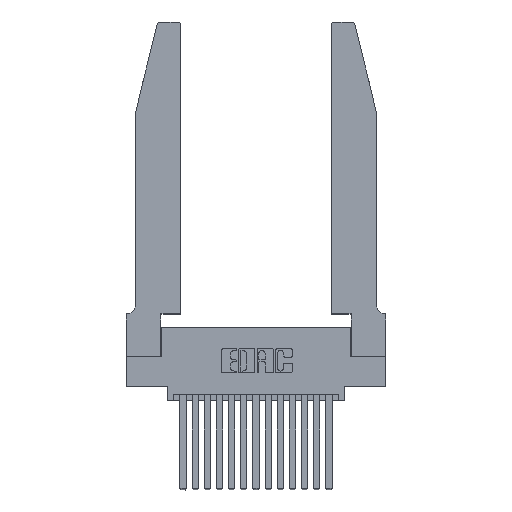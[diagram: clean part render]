
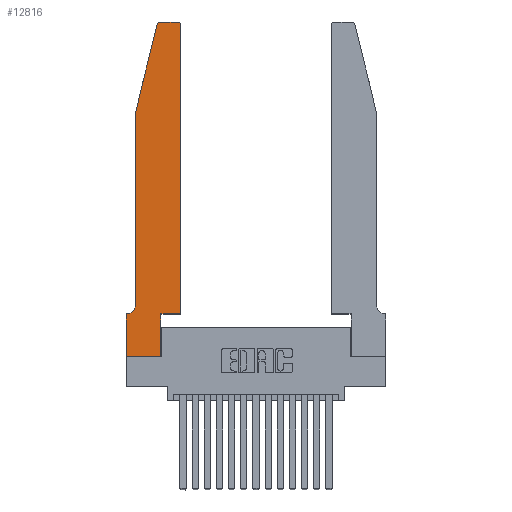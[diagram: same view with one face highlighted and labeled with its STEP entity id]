
A CAD part, top view. The second image highlights one B-rep face of the part: STEP entity #12816.
In plain terms, the highlighted planar face has unit normal (0, 0, 1).
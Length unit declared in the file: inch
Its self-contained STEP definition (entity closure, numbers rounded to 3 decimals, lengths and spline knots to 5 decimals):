
#47 = ORIENTED_EDGE ( 'NONE', *, *, #8778, .T. ) ;
#226 = LINE ( 'NONE', #14997, #3623 ) ;
#280 = VECTOR ( 'NONE', #14104, 39.37008 ) ;
#457 = DIRECTION ( 'NONE',  ( 0., 1., 0. ) ) ;
#633 = CARTESIAN_POINT ( 'NONE',  ( 0.0755, 0.35, 0.37 ) ) ;
#1047 = DIRECTION ( 'NONE',  ( 1., 0., 0. ) ) ;
#1264 = CARTESIAN_POINT ( 'NONE',  ( 0.0755, 2., 0.37 ) ) ;
#1401 = LINE ( 'NONE', #5710, #7119 ) ;
#1420 = EDGE_CURVE ( 'NONE', #13402, #14783, #5633, .T. ) ;
#1527 = EDGE_CURVE ( 'NONE', #6601, #16850, #15638, .T. ) ;
#1724 = ORIENTED_EDGE ( 'NONE', *, *, #17017, .T. ) ;
#1955 = DIRECTION ( 'NONE',  ( 1., 0., 0. ) ) ;
#2006 = ORIENTED_EDGE ( 'NONE', *, *, #1420, .T. ) ;
#2154 = CARTESIAN_POINT ( 'NONE',  ( 0.0055, 0.42, 0.37 ) ) ;
#2495 = DIRECTION ( 'NONE',  ( -1., 0., 0. ) ) ;
#2535 = AXIS2_PLACEMENT_3D ( 'NONE', #2154, #5106, #16919 ) ;
#2571 = LINE ( 'NONE', #15739, #7391 ) ;
#2753 = EDGE_CURVE ( 'NONE', #9355, #13402, #16266, .T. ) ;
#2881 = DIRECTION ( 'NONE',  ( 0., -1., 0. ) ) ;
#3074 = CARTESIAN_POINT ( 'NONE',  ( 0., 0., 0.37 ) ) ;
#3121 = ORIENTED_EDGE ( 'NONE', *, *, #12940, .T. ) ;
#3542 = DIRECTION ( 'NONE',  ( -1., 0., 0. ) ) ;
#3623 = VECTOR ( 'NONE', #1955, 39.37008 ) ;
#3868 = VERTEX_POINT ( 'NONE', #18828 ) ;
#3893 = CARTESIAN_POINT ( 'NONE',  ( 0., 0.35, 0.37 ) ) ;
#3898 = CARTESIAN_POINT ( 'NONE',  ( 0.0755, 0.42, 0.37 ) ) ;
#3967 = CARTESIAN_POINT ( 'NONE',  ( 0.0755, 2., 0.37 ) ) ;
#4467 = EDGE_CURVE ( 'NONE', #14783, #17610, #13930, .T. ) ;
#4891 = VECTOR ( 'NONE', #10074, 39.37008 ) ;
#5106 = DIRECTION ( 'NONE',  ( 0., 0., -1. ) ) ;
#5339 = CARTESIAN_POINT ( 'NONE',  ( 0.2865, 0.35, 0.37 ) ) ;
#5503 = VERTEX_POINT ( 'NONE', #17672 ) ;
#5603 = CARTESIAN_POINT ( 'NONE',  ( 0.284, 2.72, 0.37 ) ) ;
#5610 = EDGE_CURVE ( 'NONE', #18834, #8121, #226, .T. ) ;
#5633 = CIRCLE ( 'NONE', #2535, 0.07 ) ;
#5706 = DIRECTION ( 'NONE',  ( 0., 0., 1. ) ) ;
#5710 = CARTESIAN_POINT ( 'NONE',  ( 0.4505, 0.35, 0.37 ) ) ;
#6427 = VECTOR ( 'NONE', #3542, 39.37008 ) ;
#6445 = ORIENTED_EDGE ( 'NONE', *, *, #10092, .T. ) ;
#6601 = VERTEX_POINT ( 'NONE', #18458 ) ;
#6983 = PLANE ( 'NONE',  #14503 ) ;
#7119 = VECTOR ( 'NONE', #7370, 39.37008 ) ;
#7370 = DIRECTION ( 'NONE',  ( 1., 0., 0. ) ) ;
#7391 = VECTOR ( 'NONE', #2495, 39.37008 ) ;
#7796 = LINE ( 'NONE', #5339, #280 ) ;
#8121 = VERTEX_POINT ( 'NONE', #18257 ) ;
#8778 = EDGE_CURVE ( 'NONE', #14904, #9355, #9441, .T. ) ;
#9355 = VERTEX_POINT ( 'NONE', #13224 ) ;
#9441 = LINE ( 'NONE', #1264, #4891 ) ;
#9478 = LINE ( 'NONE', #16235, #12221 ) ;
#9668 = CIRCLE ( 'NONE', #12299, 0.03 ) ;
#9908 = EDGE_LOOP ( 'NONE', ( #15488, #10284, #47, #12953, #2006, #14890, #6445, #16651, #17901, #3121, #1724, #12634 ) ) ;
#10019 = AXIS2_PLACEMENT_3D ( 'NONE', #14404, #5706, #10046 ) ;
#10046 = DIRECTION ( 'NONE',  ( 1., 0., 0. ) ) ;
#10074 = DIRECTION ( 'NONE',  ( -0.239, -0.971, 0. ) ) ;
#10092 = EDGE_CURVE ( 'NONE', #17610, #18834, #16927, .T. ) ;
#10284 = ORIENTED_EDGE ( 'NONE', *, *, #18059, .T. ) ;
#10955 = EDGE_CURVE ( 'NONE', #8121, #3868, #7796, .T. ) ;
#11226 = FACE_OUTER_BOUND ( 'NONE', #9908, .T. ) ;
#11599 = CARTESIAN_POINT ( 'NONE',  ( 0.25487, 2.72718, 0.37 ) ) ;
#12112 = CARTESIAN_POINT ( 'NONE',  ( 0., 0., 0.37 ) ) ;
#12221 = VECTOR ( 'NONE', #457, 39.37008 ) ;
#12299 = AXIS2_PLACEMENT_3D ( 'NONE', #5603, #17232, #14432 ) ;
#12634 = ORIENTED_EDGE ( 'NONE', *, *, #1527, .T. ) ;
#12816 = ADVANCED_FACE ( 'NONE', ( #11226 ), #6983, .T. ) ;
#12940 = EDGE_CURVE ( 'NONE', #3868, #5503, #1401, .T. ) ;
#12953 = ORIENTED_EDGE ( 'NONE', *, *, #2753, .T. ) ;
#13092 = VECTOR ( 'NONE', #14648, 39.37008 ) ;
#13224 = CARTESIAN_POINT ( 'NONE',  ( 0.0755, 2., 0.37 ) ) ;
#13402 = VERTEX_POINT ( 'NONE', #3898 ) ;
#13930 = LINE ( 'NONE', #633, #6427 ) ;
#14104 = DIRECTION ( 'NONE',  ( 0., 1., 0. ) ) ;
#14404 = CARTESIAN_POINT ( 'NONE',  ( 0.4205, 2.72, 0.37 ) ) ;
#14432 = DIRECTION ( 'NONE',  ( 1., 0., 0. ) ) ;
#14503 = AXIS2_PLACEMENT_3D ( 'NONE', #17209, #17076, #1047 ) ;
#14648 = DIRECTION ( 'NONE',  ( 0., -1., 0. ) ) ;
#14763 = VERTEX_POINT ( 'NONE', #18395 ) ;
#14783 = VERTEX_POINT ( 'NONE', #15697 ) ;
#14890 = ORIENTED_EDGE ( 'NONE', *, *, #4467, .T. ) ;
#14904 = VERTEX_POINT ( 'NONE', #11599 ) ;
#14997 = CARTESIAN_POINT ( 'NONE',  ( 0., 0., 0.37 ) ) ;
#15488 = ORIENTED_EDGE ( 'NONE', *, *, #18580, .T. ) ;
#15638 = CIRCLE ( 'NONE', #10019, 0.03 ) ;
#15697 = CARTESIAN_POINT ( 'NONE',  ( 0.0055, 0.35, 0.37 ) ) ;
#15739 = CARTESIAN_POINT ( 'NONE',  ( 0.2605, 2.75, 0.37 ) ) ;
#16235 = CARTESIAN_POINT ( 'NONE',  ( 0.4505, 0.35, 0.37 ) ) ;
#16266 = LINE ( 'NONE', #3967, #16712 ) ;
#16651 = ORIENTED_EDGE ( 'NONE', *, *, #5610, .T. ) ;
#16712 = VECTOR ( 'NONE', #2881, 39.37008 ) ;
#16850 = VERTEX_POINT ( 'NONE', #17322 ) ;
#16919 = DIRECTION ( 'NONE',  ( -1., 0., 0. ) ) ;
#16927 = LINE ( 'NONE', #3074, #13092 ) ;
#17017 = EDGE_CURVE ( 'NONE', #5503, #6601, #9478, .T. ) ;
#17076 = DIRECTION ( 'NONE',  ( 0., 0., 1. ) ) ;
#17209 = CARTESIAN_POINT ( 'NONE',  ( 0., 0.35, 0.37 ) ) ;
#17232 = DIRECTION ( 'NONE',  ( 0., 0., 1. ) ) ;
#17322 = CARTESIAN_POINT ( 'NONE',  ( 0.4205, 2.75, 0.37 ) ) ;
#17610 = VERTEX_POINT ( 'NONE', #3893 ) ;
#17672 = CARTESIAN_POINT ( 'NONE',  ( 0.4505, 0.35, 0.37 ) ) ;
#17901 = ORIENTED_EDGE ( 'NONE', *, *, #10955, .T. ) ;
#18059 = EDGE_CURVE ( 'NONE', #14763, #14904, #9668, .T. ) ;
#18257 = CARTESIAN_POINT ( 'NONE',  ( 0.2865, 0., 0.37 ) ) ;
#18395 = CARTESIAN_POINT ( 'NONE',  ( 0.284, 2.75, 0.37 ) ) ;
#18458 = CARTESIAN_POINT ( 'NONE',  ( 0.4505, 2.72, 0.37 ) ) ;
#18580 = EDGE_CURVE ( 'NONE', #16850, #14763, #2571, .T. ) ;
#18828 = CARTESIAN_POINT ( 'NONE',  ( 0.2865, 0.35, 0.37 ) ) ;
#18834 = VERTEX_POINT ( 'NONE', #12112 ) ;
